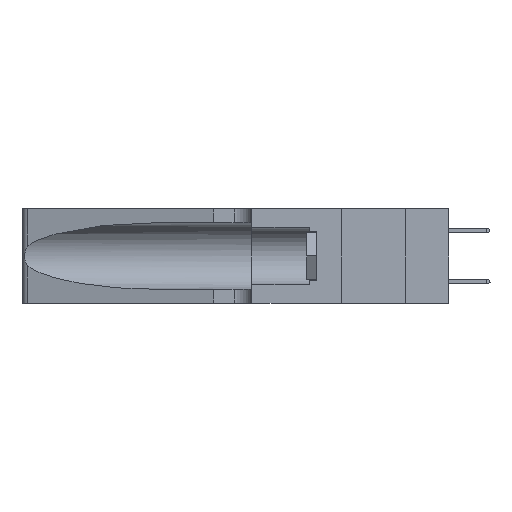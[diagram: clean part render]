
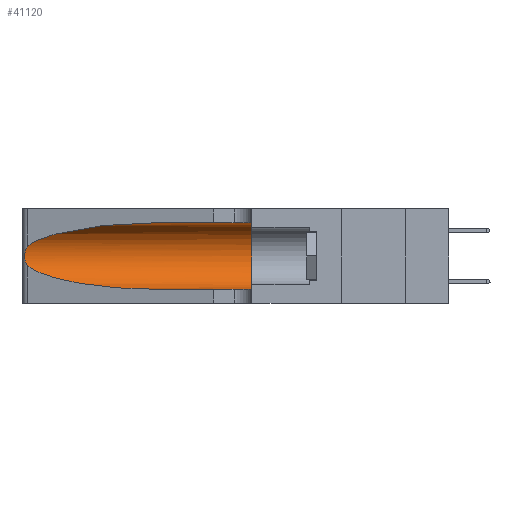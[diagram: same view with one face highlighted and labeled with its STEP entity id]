
A CAD part, left-side view. The second image highlights one B-rep face of the part: STEP entity #41120.
In plain terms, the highlighted cylindrical face has radius 3.308 mm (diameter 6.617 mm), a partial arc.
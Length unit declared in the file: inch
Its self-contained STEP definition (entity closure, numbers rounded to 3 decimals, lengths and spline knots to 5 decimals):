
#1992 = EDGE_CURVE ( 'NONE', #35736, #24601, #35026, .T. ) ;
#2481 = CARTESIAN_POINT ( 'NONE',  ( 0.1305, 0.72297, 0.31525 ) ) ;
#2643 = CARTESIAN_POINT ( 'NONE',  ( 0.25639, 1.23184, 0.21858 ) ) ;
#3357 = VERTEX_POINT ( 'NONE', #27263 ) ;
#4229 = EDGE_LOOP ( 'NONE', ( #27142, #9424, #42073, #20352, #28835, #22717 ) ) ;
#4759 = CARTESIAN_POINT ( 'NONE',  ( 0.1305, 0.35, 0.05475 ) ) ;
#4934 = CIRCLE ( 'NONE', #25536, 0.13025 ) ;
#6150 = CARTESIAN_POINT ( 'NONE',  ( 0.25487, 1.22718, 0.22369 ) ) ;
#8352 = CARTESIAN_POINT ( 'NONE',  ( 0.1305, 1.61858, 0.31525 ) ) ;
#9111 = CARTESIAN_POINT ( 'NONE',  ( 0.25487, 1.22718, 0.22369 ) ) ;
#9424 = ORIENTED_EDGE ( 'NONE', *, *, #38214, .T. ) ;
#9593 = DIRECTION ( 'NONE',  ( 0., -1., 0. ) ) ;
#10117 = VERTEX_POINT ( 'NONE', #29261 ) ;
#11839 = CYLINDRICAL_SURFACE ( 'NONE', #18603, 0.13025 ) ;
#12608 = CARTESIAN_POINT ( 'NONE',  ( 0.1305, 0.35, 0.185 ) ) ;
#12952 = CARTESIAN_POINT ( 'NONE',  ( 0.25555, 1.22993, 0.14849 ) ) ;
#13933 = FACE_OUTER_BOUND ( 'NONE', #4229, .T. ) ;
#15410 = CARTESIAN_POINT ( 'NONE',  ( 0.1305, 0.72297, 0.05475 ) ) ;
#15869 = EDGE_CURVE ( 'NONE', #26212, #41826, #42862, .T. ) ;
#15872 = VECTOR ( 'NONE', #9593, 39.37008 ) ;
#16202 = CARTESIAN_POINT ( 'NONE',  ( 0.25854, 1.2359, 0.20912 ) ) ;
#16284 = DIRECTION ( 'NONE',  ( 0., 0., 1. ) ) ;
#16341 = CARTESIAN_POINT ( 'NONE',  ( 0.25487, 1.22718, 0.14631 ) ) ;
#18603 = AXIS2_PLACEMENT_3D ( 'NONE', #34489, #20693, #37423 ) ;
#20352 = ORIENTED_EDGE ( 'NONE', *, *, #15869, .T. ) ;
#20693 = DIRECTION ( 'NONE',  ( 0., -1., 0. ) ) ;
#21123 = CARTESIAN_POINT ( 'NONE',  ( 0.1305, 1.61858, 0.05475 ) ) ;
#22717 = ORIENTED_EDGE ( 'NONE', *, *, #1992, .F. ) ;
#23632 = EDGE_CURVE ( 'NONE', #24601, #41826, #4934, .T. ) ;
#24601 = VERTEX_POINT ( 'NONE', #32475 ) ;
#25126 =( BOUNDED_CURVE ( )  B_SPLINE_CURVE ( 3, ( #2481, #39154, #42387, #9111 ),
 .UNSPECIFIED., .F., .F. ) 
 B_SPLINE_CURVE_WITH_KNOTS ( ( 4, 4 ),
 ( 1.5708, 2.84003 ),
 .UNSPECIFIED. ) 
 CURVE ( )  GEOMETRIC_REPRESENTATION_ITEM ( )  RATIONAL_B_SPLINE_CURVE ( ( 1., 0.87, 0.87, 1. ) ) 
 REPRESENTATION_ITEM ( '' )  );
#25156 = CARTESIAN_POINT ( 'NONE',  ( 0.25487, 1.22718, 0.14631 ) ) ;
#25536 = AXIS2_PLACEMENT_3D ( 'NONE', #12608, #36274, #16284 ) ;
#26001 = VECTOR ( 'NONE', #37858, 39.37008 ) ;
#26212 = VERTEX_POINT ( 'NONE', #31832 ) ;
#26535 = CARTESIAN_POINT ( 'NONE',  ( 0.25856, 1.23593, 0.16098 ) ) ;
#27142 = ORIENTED_EDGE ( 'NONE', *, *, #28808, .T. ) ;
#27263 = CARTESIAN_POINT ( 'NONE',  ( 0.25487, 1.22718, 0.14631 ) ) ;
#27508 = EDGE_CURVE ( 'NONE', #3357, #26212, #27589, .T. ) ;
#27589 =( BOUNDED_CURVE ( )  B_SPLINE_CURVE ( 3, ( #25156, #42178, #35679, #15410 ),
 .UNSPECIFIED., .F., .F. ) 
 B_SPLINE_CURVE_WITH_KNOTS ( ( 4, 4 ),
 ( 3.44316, 4.71239 ),
 .UNSPECIFIED. ) 
 CURVE ( )  GEOMETRIC_REPRESENTATION_ITEM ( )  RATIONAL_B_SPLINE_CURVE ( ( 1., 0.87, 0.87, 1. ) ) 
 REPRESENTATION_ITEM ( '' )  );
#28808 = EDGE_CURVE ( 'NONE', #35736, #10117, #25126, .T. ) ;
#28835 = ORIENTED_EDGE ( 'NONE', *, *, #23632, .F. ) ;
#29261 = CARTESIAN_POINT ( 'NONE',  ( 0.25487, 1.22718, 0.22369 ) ) ;
#29819 = CARTESIAN_POINT ( 'NONE',  ( 0.25789, 1.23486, 0.15765 ) ) ;
#31832 = CARTESIAN_POINT ( 'NONE',  ( 0.1305, 0.72297, 0.05475 ) ) ;
#32219 = B_SPLINE_CURVE_WITH_KNOTS ( 'NONE', 3,
 ( #6150, #36761, #2643, #32782, #16202, #39861, #39583, #32933, #42980, #26535, #29819, #36484, #12952, #16341 ),
 .UNSPECIFIED., .F., .F.,
 ( 4, 2, 2, 2, 2, 2, 4 ),
 ( 0., 0.00027, 0.00053, 0.00107, 0.0016, 0.00187, 0.00214 ),
 .UNSPECIFIED. ) ;
#32475 = CARTESIAN_POINT ( 'NONE',  ( 0.1305, 0.35, 0.31525 ) ) ;
#32782 = CARTESIAN_POINT ( 'NONE',  ( 0.25787, 1.23484, 0.2124 ) ) ;
#32933 = CARTESIAN_POINT ( 'NONE',  ( 0.26075, 1.23896, 0.178 ) ) ;
#34489 = CARTESIAN_POINT ( 'NONE',  ( 0.1305, 1.61858, 0.185 ) ) ;
#34681 = CARTESIAN_POINT ( 'NONE',  ( 0.1305, 0.72297, 0.31525 ) ) ;
#35026 = LINE ( 'NONE', #8352, #26001 ) ;
#35679 = CARTESIAN_POINT ( 'NONE',  ( 0.18966, 0.96281, 0.05475 ) ) ;
#35736 = VERTEX_POINT ( 'NONE', #34681 ) ;
#36274 = DIRECTION ( 'NONE',  ( 0., 1., 0. ) ) ;
#36484 = CARTESIAN_POINT ( 'NONE',  ( 0.25639, 1.23186, 0.15144 ) ) ;
#36761 = CARTESIAN_POINT ( 'NONE',  ( 0.25555, 1.22994, 0.2215 ) ) ;
#37423 = DIRECTION ( 'NONE',  ( 0., 0., -1. ) ) ;
#37858 = DIRECTION ( 'NONE',  ( 0., -1., 0. ) ) ;
#38214 = EDGE_CURVE ( 'NONE', #10117, #3357, #32219, .T. ) ;
#39154 = CARTESIAN_POINT ( 'NONE',  ( 0.18966, 0.96281, 0.31525 ) ) ;
#39583 = CARTESIAN_POINT ( 'NONE',  ( 0.26075, 1.23896, 0.19203 ) ) ;
#39861 = CARTESIAN_POINT ( 'NONE',  ( 0.26018, 1.23835, 0.19895 ) ) ;
#41120 = ADVANCED_FACE ( 'NONE', ( #13933 ), #11839, .F. ) ;
#41826 = VERTEX_POINT ( 'NONE', #4759 ) ;
#42073 = ORIENTED_EDGE ( 'NONE', *, *, #27508, .T. ) ;
#42178 = CARTESIAN_POINT ( 'NONE',  ( 0.2373, 1.15595, 0.08982 ) ) ;
#42387 = CARTESIAN_POINT ( 'NONE',  ( 0.2373, 1.15595, 0.28018 ) ) ;
#42862 = LINE ( 'NONE', #21123, #15872 ) ;
#42980 = CARTESIAN_POINT ( 'NONE',  ( 0.26017, 1.23833, 0.17102 ) ) ;
